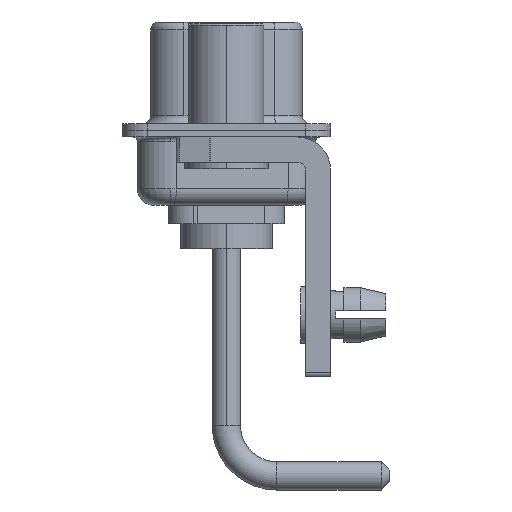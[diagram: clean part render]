
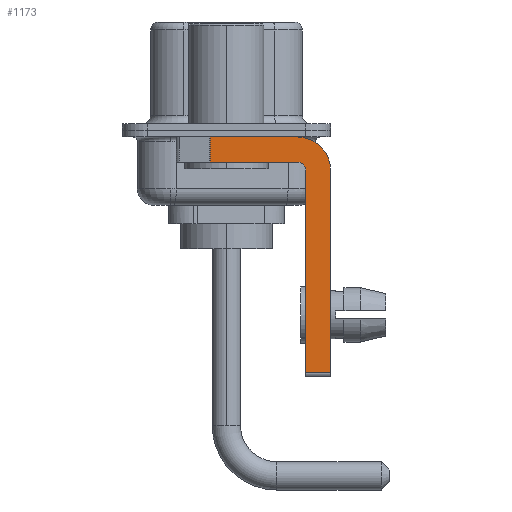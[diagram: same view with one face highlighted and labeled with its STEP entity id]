
A CAD part, left-side view. The second image highlights one B-rep face of the part: STEP entity #1173.
In plain terms, the highlighted planar face has unit normal (-1, 0, 0).
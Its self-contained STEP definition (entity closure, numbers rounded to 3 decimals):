
#241 = VERTEX_POINT ( 'NONE', #14513 ) ;
#581 = EDGE_CURVE ( 'NONE', #16845, #12404, #3738, .T. ) ;
#874 = DIRECTION ( 'NONE',  ( 0., 0., 1. ) ) ;
#955 = EDGE_LOOP ( 'NONE', ( #13462, #4002, #13400, #15823, #5437, #12343, #10596, #2088 ) ) ;
#1173 = ADVANCED_FACE ( 'NONE', ( #14964 ), #3032, .F. ) ;
#1454 = CARTESIAN_POINT ( 'NONE',  ( -2.9, 3., -0.4 ) ) ;
#1552 = LINE ( 'NONE', #1454, #19209 ) ;
#2083 = AXIS2_PLACEMENT_3D ( 'NONE', #19200, #5534, #9714 ) ;
#2088 = ORIENTED_EDGE ( 'NONE', *, *, #19007, .F. ) ;
#2345 = DIRECTION ( 'NONE',  ( 0., 0., 1. ) ) ;
#2612 = VERTEX_POINT ( 'NONE', #4799 ) ;
#2655 = LINE ( 'NONE', #13374, #11900 ) ;
#3032 = PLANE ( 'NONE',  #8470 ) ;
#3738 = LINE ( 'NONE', #15985, #18292 ) ;
#4002 = ORIENTED_EDGE ( 'NONE', *, *, #7611, .T. ) ;
#4311 = DIRECTION ( 'NONE',  ( 1., 0., 0. ) ) ;
#4425 = VECTOR ( 'NONE', #2345, 1000. ) ;
#4799 = CARTESIAN_POINT ( 'NONE',  ( -2.9, -4.75, -14.55 ) ) ;
#4964 = EDGE_CURVE ( 'NONE', #2612, #17491, #17065, .T. ) ;
#5137 = VERTEX_POINT ( 'NONE', #5785 ) ;
#5329 = AXIS2_PLACEMENT_3D ( 'NONE', #17251, #15883, #874 ) ;
#5437 = ORIENTED_EDGE ( 'NONE', *, *, #4964, .F. ) ;
#5534 = DIRECTION ( 'NONE',  ( 1., 0., 0. ) ) ;
#5781 = DIRECTION ( 'NONE',  ( 0., -1., 0. ) ) ;
#5785 = CARTESIAN_POINT ( 'NONE',  ( -2.9, 0.978, -1.9 ) ) ;
#7483 = CARTESIAN_POINT ( 'NONE',  ( -2.9, -4.25, -2.4 ) ) ;
#7611 = EDGE_CURVE ( 'NONE', #17393, #5137, #17903, .T. ) ;
#8470 = AXIS2_PLACEMENT_3D ( 'NONE', #7483, #4311, #8661 ) ;
#8661 = DIRECTION ( 'NONE',  ( 0., 0., -1. ) ) ;
#8686 = DIRECTION ( 'NONE',  ( 0., 0., -1. ) ) ;
#8722 = VECTOR ( 'NONE', #19315, 1000. ) ;
#9027 = VECTOR ( 'NONE', #18095, 1000. ) ;
#9714 = DIRECTION ( 'NONE',  ( 0., 0., -1. ) ) ;
#10596 = ORIENTED_EDGE ( 'NONE', *, *, #581, .F. ) ;
#10941 = CARTESIAN_POINT ( 'NONE',  ( -2.9, -4.75, -2.4 ) ) ;
#11900 = VECTOR ( 'NONE', #19454, 1000. ) ;
#12343 = ORIENTED_EDGE ( 'NONE', *, *, #16420, .T. ) ;
#12404 = VERTEX_POINT ( 'NONE', #19421 ) ;
#12523 = CARTESIAN_POINT ( 'NONE',  ( -2.9, -4.25, -0.4 ) ) ;
#12554 = VERTEX_POINT ( 'NONE', #12523 ) ;
#13207 = EDGE_CURVE ( 'NONE', #17491, #241, #13935, .T. ) ;
#13374 = CARTESIAN_POINT ( 'NONE',  ( -2.9, -4.25, -14.55 ) ) ;
#13400 = ORIENTED_EDGE ( 'NONE', *, *, #19265, .F. ) ;
#13462 = ORIENTED_EDGE ( 'NONE', *, *, #18341, .F. ) ;
#13516 = LINE ( 'NONE', #19595, #9027 ) ;
#13935 = CIRCLE ( 'NONE', #5329, 0.5 ) ;
#14078 = CARTESIAN_POINT ( 'NONE',  ( -2.9, -4.75, -14.8 ) ) ;
#14513 = CARTESIAN_POINT ( 'NONE',  ( -2.9, -4.25, -1.9 ) ) ;
#14964 = FACE_OUTER_BOUND ( 'NONE', #955, .T. ) ;
#15340 = CARTESIAN_POINT ( 'NONE',  ( -2.9, 0.978, -0.4 ) ) ;
#15823 = ORIENTED_EDGE ( 'NONE', *, *, #13207, .F. ) ;
#15883 = DIRECTION ( 'NONE',  ( -1., 0., 0. ) ) ;
#15985 = CARTESIAN_POINT ( 'NONE',  ( -2.9, -6.25, -2.4 ) ) ;
#16037 = CARTESIAN_POINT ( 'NONE',  ( -2.9, -6.25, -2.4 ) ) ;
#16420 = EDGE_CURVE ( 'NONE', #2612, #12404, #2655, .T. ) ;
#16845 = VERTEX_POINT ( 'NONE', #16037 ) ;
#17065 = LINE ( 'NONE', #14078, #4425 ) ;
#17251 = CARTESIAN_POINT ( 'NONE',  ( -2.9, -4.25, -2.4 ) ) ;
#17393 = VERTEX_POINT ( 'NONE', #15340 ) ;
#17491 = VERTEX_POINT ( 'NONE', #10941 ) ;
#17903 = LINE ( 'NONE', #18011, #8722 ) ;
#18011 = CARTESIAN_POINT ( 'NONE',  ( -2.9, 0.978, -1.9 ) ) ;
#18095 = DIRECTION ( 'NONE',  ( 0., 1., 0. ) ) ;
#18292 = VECTOR ( 'NONE', #8686, 1000. ) ;
#18341 = EDGE_CURVE ( 'NONE', #17393, #12554, #1552, .T. ) ;
#19007 = EDGE_CURVE ( 'NONE', #12554, #16845, #19241, .T. ) ;
#19200 = CARTESIAN_POINT ( 'NONE',  ( -2.9, -4.25, -2.4 ) ) ;
#19209 = VECTOR ( 'NONE', #5781, 1000. ) ;
#19241 = CIRCLE ( 'NONE', #2083, 2. ) ;
#19265 = EDGE_CURVE ( 'NONE', #241, #5137, #13516, .T. ) ;
#19315 = DIRECTION ( 'NONE',  ( 0., 0., -1. ) ) ;
#19421 = CARTESIAN_POINT ( 'NONE',  ( -2.9, -6.25, -14.55 ) ) ;
#19454 = DIRECTION ( 'NONE',  ( 0., -1., 0. ) ) ;
#19595 = CARTESIAN_POINT ( 'NONE',  ( -2.9, -4.25, -1.9 ) ) ;
